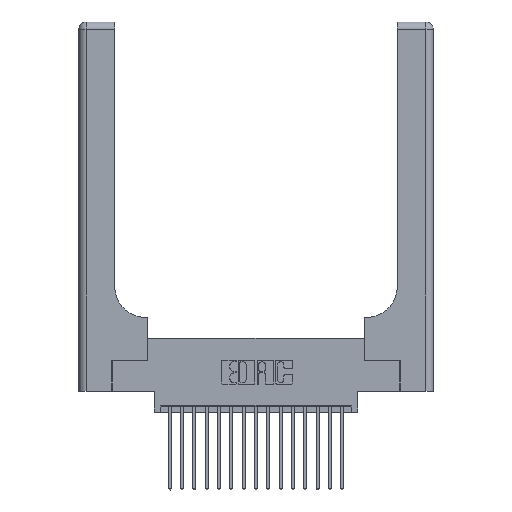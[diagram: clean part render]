
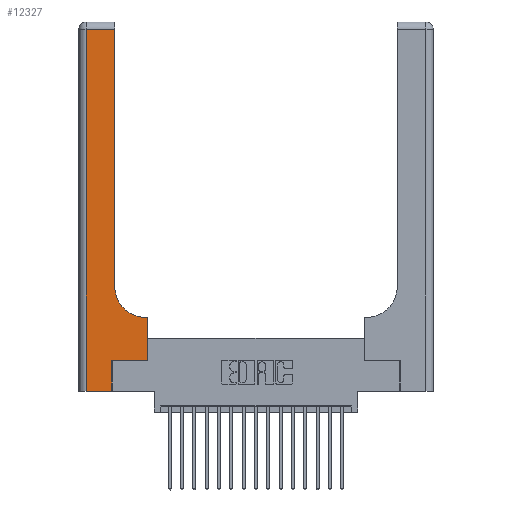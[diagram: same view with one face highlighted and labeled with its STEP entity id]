
A CAD part, top view. The second image highlights one B-rep face of the part: STEP entity #12327.
In plain terms, the highlighted planar face has unit normal (0, 0, 1).
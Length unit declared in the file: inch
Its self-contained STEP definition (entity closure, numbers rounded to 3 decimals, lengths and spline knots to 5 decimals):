
#537 = EDGE_LOOP ( 'NONE', ( #7629, #11899, #8759, #20428, #7516, #14630, #19572, #18644, #10909 ) ) ;
#884 = LINE ( 'NONE', #4574, #17436 ) ;
#1335 = CARTESIAN_POINT ( 'NONE',  ( 0.2915, 2.94, 0.37 ) ) ;
#1393 = VECTOR ( 'NONE', #14599, 39.37008 ) ;
#1655 = CIRCLE ( 'NONE', #14421, 0.25 ) ;
#1684 = EDGE_CURVE ( 'NONE', #9968, #20198, #7056, .T. ) ;
#1892 = EDGE_CURVE ( 'NONE', #17700, #6385, #17308, .T. ) ;
#2109 = EDGE_CURVE ( 'NONE', #6385, #6219, #20713, .T. ) ;
#2119 = CARTESIAN_POINT ( 'NONE',  ( 0.5585, 0.25, 0.37 ) ) ;
#2183 = DIRECTION ( 'NONE',  ( -1., 0., 0. ) ) ;
#2668 = DIRECTION ( 'NONE',  ( 0., 1., 0. ) ) ;
#3230 = CARTESIAN_POINT ( 'NONE',  ( 0.269, 0., 0.37 ) ) ;
#3551 = DIRECTION ( 'NONE',  ( -1., 0., 0. ) ) ;
#3935 = DIRECTION ( 'NONE',  ( 0., 1., 0. ) ) ;
#4521 = VECTOR ( 'NONE', #2668, 39.37008 ) ;
#4574 = CARTESIAN_POINT ( 'NONE',  ( 0.2915, 0.6, 0.37 ) ) ;
#5280 = CARTESIAN_POINT ( 'NONE',  ( 0.06, 0., 0.37 ) ) ;
#5992 = VERTEX_POINT ( 'NONE', #11069 ) ;
#6219 = VERTEX_POINT ( 'NONE', #13815 ) ;
#6385 = VERTEX_POINT ( 'NONE', #1335 ) ;
#6435 = CARTESIAN_POINT ( 'NONE',  ( 0., 0., 0.37 ) ) ;
#6551 = CARTESIAN_POINT ( 'NONE',  ( 0., 2.94, 0.37 ) ) ;
#6916 = LINE ( 'NONE', #3230, #1393 ) ;
#7056 = LINE ( 'NONE', #19846, #17559 ) ;
#7115 = CARTESIAN_POINT ( 'NONE',  ( 0.5585, 0.6, 0.37 ) ) ;
#7516 = ORIENTED_EDGE ( 'NONE', *, *, #9869, .T. ) ;
#7629 = ORIENTED_EDGE ( 'NONE', *, *, #1892, .T. ) ;
#8556 = FACE_OUTER_BOUND ( 'NONE', #537, .T. ) ;
#8759 = ORIENTED_EDGE ( 'NONE', *, *, #10445, .T. ) ;
#8769 = CARTESIAN_POINT ( 'NONE',  ( 0.2915, 0.85, 0.37 ) ) ;
#9370 = VECTOR ( 'NONE', #12846, 39.37008 ) ;
#9400 = LINE ( 'NONE', #14320, #17657 ) ;
#9453 = VERTEX_POINT ( 'NONE', #5280 ) ;
#9869 = EDGE_CURVE ( 'NONE', #12973, #9968, #6916, .T. ) ;
#9955 = CARTESIAN_POINT ( 'NONE',  ( 0., 3., 0.37 ) ) ;
#9960 = VERTEX_POINT ( 'NONE', #7115 ) ;
#9968 = VERTEX_POINT ( 'NONE', #13236 ) ;
#10264 = DIRECTION ( 'NONE',  ( 1., 0., 0. ) ) ;
#10445 = EDGE_CURVE ( 'NONE', #6219, #9453, #9400, .T. ) ;
#10748 = LINE ( 'NONE', #18369, #12482 ) ;
#10909 = ORIENTED_EDGE ( 'NONE', *, *, #15659, .T. ) ;
#11069 = CARTESIAN_POINT ( 'NONE',  ( 0.5415, 0.6, 0.37 ) ) ;
#11232 = CARTESIAN_POINT ( 'NONE',  ( 0.5415, 0.85, 0.37 ) ) ;
#11899 = ORIENTED_EDGE ( 'NONE', *, *, #2109, .T. ) ;
#12327 = ADVANCED_FACE ( 'NONE', ( #8556 ), #16459, .F. ) ;
#12482 = VECTOR ( 'NONE', #3935, 39.37008 ) ;
#12846 = DIRECTION ( 'NONE',  ( 1., 0., 0. ) ) ;
#12886 = DIRECTION ( 'NONE',  ( 0., -1., 0. ) ) ;
#12933 = CARTESIAN_POINT ( 'NONE',  ( 0.269, 0., 0.37 ) ) ;
#12947 = DIRECTION ( 'NONE',  ( 0., 0., -1. ) ) ;
#12973 = VERTEX_POINT ( 'NONE', #12933 ) ;
#13236 = CARTESIAN_POINT ( 'NONE',  ( 0.269, 0.25, 0.37 ) ) ;
#13614 = LINE ( 'NONE', #6435, #9370 ) ;
#13815 = CARTESIAN_POINT ( 'NONE',  ( 0.06, 2.94, 0.37 ) ) ;
#13889 = CARTESIAN_POINT ( 'NONE',  ( 0.2915, 3., 0.37 ) ) ;
#14040 = DIRECTION ( 'NONE',  ( -1., 0., 0. ) ) ;
#14320 = CARTESIAN_POINT ( 'NONE',  ( 0.06, 3., 0.37 ) ) ;
#14421 = AXIS2_PLACEMENT_3D ( 'NONE', #11232, #12947, #14650 ) ;
#14599 = DIRECTION ( 'NONE',  ( 0., 1., 0. ) ) ;
#14630 = ORIENTED_EDGE ( 'NONE', *, *, #1684, .T. ) ;
#14650 = DIRECTION ( 'NONE',  ( 1., 0., 0. ) ) ;
#14945 = DIRECTION ( 'NONE',  ( 0., 0., -1. ) ) ;
#15363 = EDGE_CURVE ( 'NONE', #20198, #9960, #10748, .T. ) ;
#15659 = EDGE_CURVE ( 'NONE', #5992, #17700, #1655, .T. ) ;
#16459 = PLANE ( 'NONE',  #19470 ) ;
#17308 = LINE ( 'NONE', #13889, #4521 ) ;
#17318 = EDGE_CURVE ( 'NONE', #9960, #5992, #884, .T. ) ;
#17436 = VECTOR ( 'NONE', #14040, 39.37008 ) ;
#17559 = VECTOR ( 'NONE', #10264, 39.37008 ) ;
#17657 = VECTOR ( 'NONE', #12886, 39.37008 ) ;
#17700 = VERTEX_POINT ( 'NONE', #8769 ) ;
#17961 = VECTOR ( 'NONE', #3551, 39.37008 ) ;
#18369 = CARTESIAN_POINT ( 'NONE',  ( 0.5585, 0.25, 0.37 ) ) ;
#18641 = EDGE_CURVE ( 'NONE', #9453, #12973, #13614, .T. ) ;
#18644 = ORIENTED_EDGE ( 'NONE', *, *, #17318, .T. ) ;
#19470 = AXIS2_PLACEMENT_3D ( 'NONE', #9955, #14945, #2183 ) ;
#19572 = ORIENTED_EDGE ( 'NONE', *, *, #15363, .T. ) ;
#19846 = CARTESIAN_POINT ( 'NONE',  ( 0.269, 0.25, 0.37 ) ) ;
#20198 = VERTEX_POINT ( 'NONE', #2119 ) ;
#20428 = ORIENTED_EDGE ( 'NONE', *, *, #18641, .T. ) ;
#20713 = LINE ( 'NONE', #6551, #17961 ) ;
